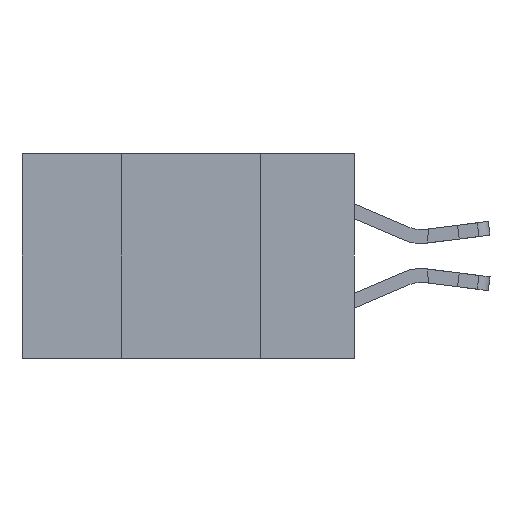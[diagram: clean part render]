
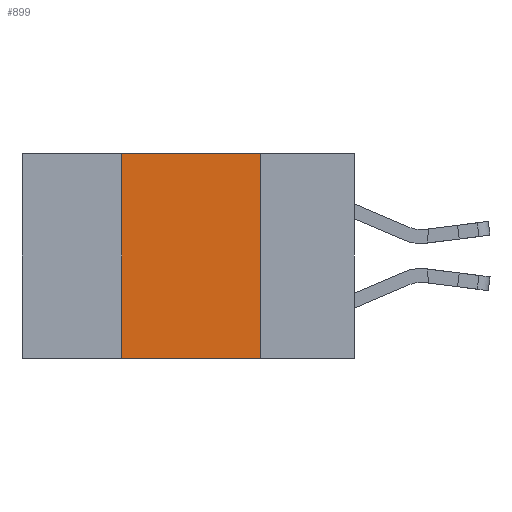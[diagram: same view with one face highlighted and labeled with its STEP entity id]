
A CAD part, left-side view. The second image highlights one B-rep face of the part: STEP entity #899.
In plain terms, the highlighted planar face has unit normal (-1, 0, 0).
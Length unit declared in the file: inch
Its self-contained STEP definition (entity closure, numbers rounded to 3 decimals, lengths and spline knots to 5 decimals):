
#556 = EDGE_CURVE ( 'NONE', #7876, #6620, #12301, .T. ) ;
#563 = VERTEX_POINT ( 'NONE', #9785 ) ;
#899 = ADVANCED_FACE ( 'NONE', ( #13551 ), #10941, .F. ) ;
#1095 = VECTOR ( 'NONE', #7308, 39.37008 ) ;
#1334 = DIRECTION ( 'NONE',  ( 0., -1., 0. ) ) ;
#1502 = CARTESIAN_POINT ( 'NONE',  ( 0., 0.6, -0.37 ) ) ;
#1517 = ORIENTED_EDGE ( 'NONE', *, *, #556, .F. ) ;
#1575 = EDGE_CURVE ( 'NONE', #6620, #4687, #10345, .T. ) ;
#1677 = ORIENTED_EDGE ( 'NONE', *, *, #1575, .F. ) ;
#1714 = ORIENTED_EDGE ( 'NONE', *, *, #2109, .F. ) ;
#2109 = EDGE_CURVE ( 'NONE', #563, #7876, #5096, .T. ) ;
#2519 = CARTESIAN_POINT ( 'NONE',  ( 0., 0.17, -0.37 ) ) ;
#2878 = EDGE_CURVE ( 'NONE', #563, #4687, #6476, .T. ) ;
#3601 = ORIENTED_EDGE ( 'NONE', *, *, #2878, .T. ) ;
#3720 = CARTESIAN_POINT ( 'NONE',  ( 0., 0.17, -0.37 ) ) ;
#4687 = VERTEX_POINT ( 'NONE', #3720 ) ;
#4745 = VECTOR ( 'NONE', #13877, 39.37008 ) ;
#4912 = CARTESIAN_POINT ( 'NONE',  ( 0., 0.42, 0. ) ) ;
#5096 = LINE ( 'NONE', #11335, #4745 ) ;
#6109 = VECTOR ( 'NONE', #1334, 39.37008 ) ;
#6474 = DIRECTION ( 'NONE',  ( 1., 0., 0. ) ) ;
#6476 = LINE ( 'NONE', #1502, #6109 ) ;
#6620 = VERTEX_POINT ( 'NONE', #11072 ) ;
#7308 = DIRECTION ( 'NONE',  ( 0., 0., -1. ) ) ;
#7876 = VERTEX_POINT ( 'NONE', #4912 ) ;
#9785 = CARTESIAN_POINT ( 'NONE',  ( 0., 0.42, -0.37 ) ) ;
#9974 = DIRECTION ( 'NONE',  ( 0., -1., 0. ) ) ;
#10345 = LINE ( 'NONE', #2519, #1095 ) ;
#10941 = PLANE ( 'NONE',  #14328 ) ;
#11072 = CARTESIAN_POINT ( 'NONE',  ( 0., 0.17, 0. ) ) ;
#11335 = CARTESIAN_POINT ( 'NONE',  ( 0., 0.42, -0.37 ) ) ;
#11808 = CARTESIAN_POINT ( 'NONE',  ( 0., 0.6, 0. ) ) ;
#12301 = LINE ( 'NONE', #12920, #14634 ) ;
#12920 = CARTESIAN_POINT ( 'NONE',  ( 0., 0.6, 0. ) ) ;
#13478 = DIRECTION ( 'NONE',  ( 0., 0., -1. ) ) ;
#13551 = FACE_OUTER_BOUND ( 'NONE', #13641, .T. ) ;
#13641 = EDGE_LOOP ( 'NONE', ( #1677, #1517, #1714, #3601 ) ) ;
#13877 = DIRECTION ( 'NONE',  ( 0., 0., 1. ) ) ;
#14328 = AXIS2_PLACEMENT_3D ( 'NONE', #11808, #6474, #13478 ) ;
#14634 = VECTOR ( 'NONE', #9974, 39.37008 ) ;
